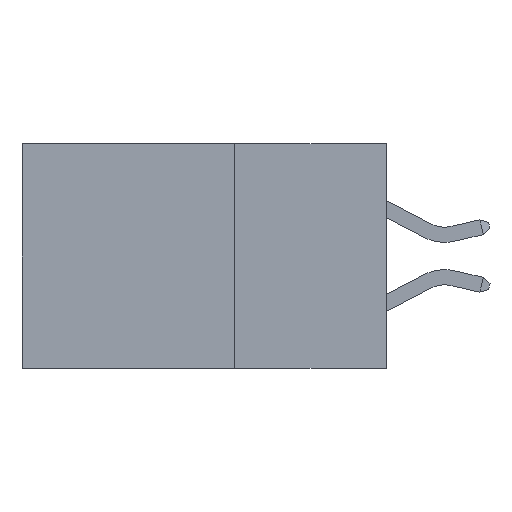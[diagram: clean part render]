
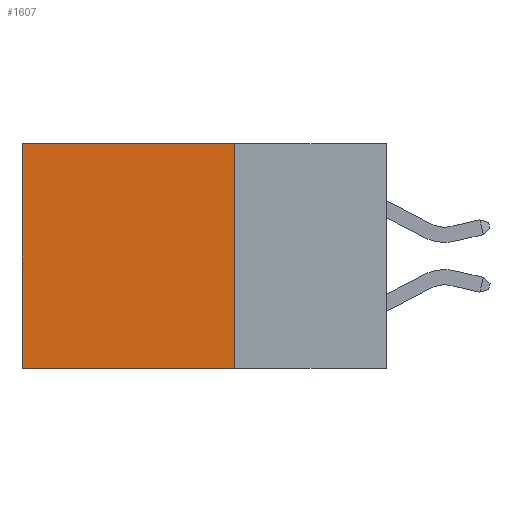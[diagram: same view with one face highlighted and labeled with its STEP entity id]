
A CAD part, left-side view. The second image highlights one B-rep face of the part: STEP entity #1607.
In plain terms, the highlighted planar face has unit normal (-1, 0, 0).
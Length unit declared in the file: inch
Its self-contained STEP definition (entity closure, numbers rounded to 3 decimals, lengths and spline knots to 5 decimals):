
#60 = CARTESIAN_POINT ( 'NONE',  ( 0.2615, 0.25, 0. ) ) ;
#135 = LINE ( 'NONE', #2320, #8990 ) ;
#565 = VERTEX_POINT ( 'NONE', #9228 ) ;
#755 = EDGE_CURVE ( 'NONE', #10604, #565, #4251, .T. ) ;
#845 = EDGE_LOOP ( 'NONE', ( #7006, #3176, #1335, #1759 ) ) ;
#1335 = ORIENTED_EDGE ( 'NONE', *, *, #3539, .F. ) ;
#1607 = ADVANCED_FACE ( 'NONE', ( #7251 ), #9694, .F. ) ;
#1729 = CARTESIAN_POINT ( 'NONE',  ( 0.2615, 0.25, -0.37 ) ) ;
#1759 = ORIENTED_EDGE ( 'NONE', *, *, #755, .T. ) ;
#2212 = AXIS2_PLACEMENT_3D ( 'NONE', #9740, #9651, #9635 ) ;
#2320 = CARTESIAN_POINT ( 'NONE',  ( 0.2615, 0.25, -0.37 ) ) ;
#3176 = ORIENTED_EDGE ( 'NONE', *, *, #6904, .F. ) ;
#3193 = VERTEX_POINT ( 'NONE', #1729 ) ;
#3539 = EDGE_CURVE ( 'NONE', #10604, #3193, #10450, .T. ) ;
#4251 = LINE ( 'NONE', #7449, #10569 ) ;
#5067 = CARTESIAN_POINT ( 'NONE',  ( 0.2615, 0.6, -0.37 ) ) ;
#5783 = DIRECTION ( 'NONE',  ( 0., 1., 0. ) ) ;
#5891 = DIRECTION ( 'NONE',  ( 0., 0., -1. ) ) ;
#6640 = LINE ( 'NONE', #5067, #10738 ) ;
#6904 = EDGE_CURVE ( 'NONE', #3193, #7052, #135, .T. ) ;
#7006 = ORIENTED_EDGE ( 'NONE', *, *, #8277, .T. ) ;
#7052 = VERTEX_POINT ( 'NONE', #9311 ) ;
#7251 = FACE_OUTER_BOUND ( 'NONE', #845, .T. ) ;
#7295 = DIRECTION ( 'NONE',  ( 0., 1., 0. ) ) ;
#7449 = CARTESIAN_POINT ( 'NONE',  ( 0.2615, 0.25, 0. ) ) ;
#8059 = VECTOR ( 'NONE', #9963, 39.37008 ) ;
#8277 = EDGE_CURVE ( 'NONE', #565, #7052, #6640, .T. ) ;
#8990 = VECTOR ( 'NONE', #5783, 39.37008 ) ;
#9228 = CARTESIAN_POINT ( 'NONE',  ( 0.2615, 0.6, 0. ) ) ;
#9311 = CARTESIAN_POINT ( 'NONE',  ( 0.2615, 0.6, -0.37 ) ) ;
#9635 = DIRECTION ( 'NONE',  ( 0., 0., -1. ) ) ;
#9651 = DIRECTION ( 'NONE',  ( 1., 0., 0. ) ) ;
#9694 = PLANE ( 'NONE',  #2212 ) ;
#9740 = CARTESIAN_POINT ( 'NONE',  ( 0.2615, 0.25, -0.37 ) ) ;
#9963 = DIRECTION ( 'NONE',  ( 0., 0., -1. ) ) ;
#10339 = CARTESIAN_POINT ( 'NONE',  ( 0.2615, 0.25, -0.37 ) ) ;
#10450 = LINE ( 'NONE', #10339, #8059 ) ;
#10569 = VECTOR ( 'NONE', #7295, 39.37008 ) ;
#10604 = VERTEX_POINT ( 'NONE', #60 ) ;
#10738 = VECTOR ( 'NONE', #5891, 39.37008 ) ;
